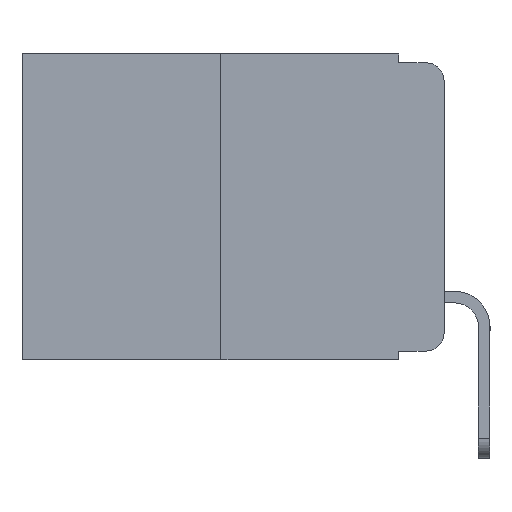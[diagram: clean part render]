
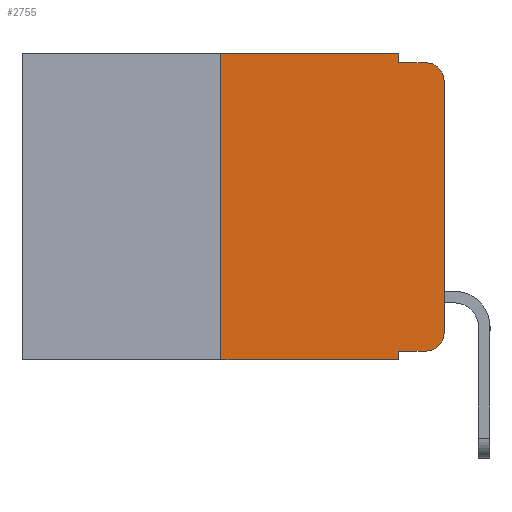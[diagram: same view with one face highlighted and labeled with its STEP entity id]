
A CAD part, left-side view. The second image highlights one B-rep face of the part: STEP entity #2755.
In plain terms, the highlighted planar face has unit normal (-1, 0, 0).
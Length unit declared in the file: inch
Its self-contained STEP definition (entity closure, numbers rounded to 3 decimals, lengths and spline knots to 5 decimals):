
#52 = EDGE_LOOP ( 'NONE', ( #12874, #5907, #13271, #6092, #5603, #7605, #6433, #11497, #13765, #5686 ) ) ;
#112 = DIRECTION ( 'NONE',  ( 0., -1., 0. ) ) ;
#180 = DIRECTION ( 'NONE',  ( -1., 0., 0. ) ) ;
#363 = VERTEX_POINT ( 'NONE', #12817 ) ;
#696 = VERTEX_POINT ( 'NONE', #8102 ) ;
#709 = DIRECTION ( 'NONE',  ( 0., 0., 1. ) ) ;
#1268 = DIRECTION ( 'NONE',  ( 0., 0., -1. ) ) ;
#1336 = CIRCLE ( 'NONE', #10804, 0.02 ) ;
#1537 = VECTOR ( 'NONE', #11410, 39.37008 ) ;
#1791 = VECTOR ( 'NONE', #3178, 39.37008 ) ;
#1844 = CARTESIAN_POINT ( 'NONE',  ( 0., 0.25, 0. ) ) ;
#2225 = VECTOR ( 'NONE', #6488, 39.37008 ) ;
#2282 = VERTEX_POINT ( 'NONE', #8865 ) ;
#2755 = ADVANCED_FACE ( 'NONE', ( #12239 ), #7552, .F. ) ;
#2836 = VERTEX_POINT ( 'NONE', #5837 ) ;
#3178 = DIRECTION ( 'NONE',  ( 0., -1., 0. ) ) ;
#3479 = VERTEX_POINT ( 'NONE', #12626 ) ;
#3719 = CARTESIAN_POINT ( 'NONE',  ( 0., 0.25, -0.343 ) ) ;
#3824 = VERTEX_POINT ( 'NONE', #12003 ) ;
#4120 = CIRCLE ( 'NONE', #6635, 0.02 ) ;
#4322 = AXIS2_PLACEMENT_3D ( 'NONE', #6410, #10486, #1268 ) ;
#4832 = CARTESIAN_POINT ( 'NONE',  ( 0., 0.25, 0. ) ) ;
#5000 = LINE ( 'NONE', #8538, #1791 ) ;
#5401 = CARTESIAN_POINT ( 'NONE',  ( 0., 0.051, 0. ) ) ;
#5542 = CARTESIAN_POINT ( 'NONE',  ( 0., 0.02, -0.03 ) ) ;
#5603 = ORIENTED_EDGE ( 'NONE', *, *, #14523, .F. ) ;
#5686 = ORIENTED_EDGE ( 'NONE', *, *, #11915, .T. ) ;
#5837 = CARTESIAN_POINT ( 'NONE',  ( 0., 0., -0.313 ) ) ;
#5885 = VERTEX_POINT ( 'NONE', #7036 ) ;
#5907 = ORIENTED_EDGE ( 'NONE', *, *, #12143, .T. ) ;
#6092 = ORIENTED_EDGE ( 'NONE', *, *, #12069, .F. ) ;
#6410 = CARTESIAN_POINT ( 'NONE',  ( 0., 0.473, 0. ) ) ;
#6433 = ORIENTED_EDGE ( 'NONE', *, *, #13144, .T. ) ;
#6488 = DIRECTION ( 'NONE',  ( 0., 0., -1. ) ) ;
#6495 = LINE ( 'NONE', #10785, #14507 ) ;
#6615 = DIRECTION ( 'NONE',  ( 0., 0., -1. ) ) ;
#6635 = AXIS2_PLACEMENT_3D ( 'NONE', #7350, #180, #8441 ) ;
#6946 = LINE ( 'NONE', #12173, #10099 ) ;
#7036 = CARTESIAN_POINT ( 'NONE',  ( 0., 0.051, -0.333 ) ) ;
#7205 = CARTESIAN_POINT ( 'NONE',  ( 0., 0.473, 0. ) ) ;
#7350 = CARTESIAN_POINT ( 'NONE',  ( 0., 0.02, -0.313 ) ) ;
#7552 = PLANE ( 'NONE',  #4322 ) ;
#7605 = ORIENTED_EDGE ( 'NONE', *, *, #12067, .F. ) ;
#8019 = DIRECTION ( 'NONE',  ( 0., -1., 0. ) ) ;
#8102 = CARTESIAN_POINT ( 'NONE',  ( 0., 0.051, -0.343 ) ) ;
#8165 = LINE ( 'NONE', #5401, #2225 ) ;
#8441 = DIRECTION ( 'NONE',  ( 0., 0., -1. ) ) ;
#8490 = VECTOR ( 'NONE', #10625, 39.37008 ) ;
#8538 = CARTESIAN_POINT ( 'NONE',  ( 0., 0.051, -0.01 ) ) ;
#8814 = VERTEX_POINT ( 'NONE', #4832 ) ;
#8865 = CARTESIAN_POINT ( 'NONE',  ( 0., 0., -0.03 ) ) ;
#9147 = VECTOR ( 'NONE', #13629, 39.37008 ) ;
#9493 = VECTOR ( 'NONE', #112, 39.37008 ) ;
#9953 = VERTEX_POINT ( 'NONE', #3719 ) ;
#10099 = VECTOR ( 'NONE', #8019, 39.37008 ) ;
#10387 = LINE ( 'NONE', #7205, #1537 ) ;
#10486 = DIRECTION ( 'NONE',  ( 1., 0., 0. ) ) ;
#10625 = DIRECTION ( 'NONE',  ( 0., 0., 1. ) ) ;
#10785 = CARTESIAN_POINT ( 'NONE',  ( 0., 0., 0. ) ) ;
#10804 = AXIS2_PLACEMENT_3D ( 'NONE', #5542, #12816, #6615 ) ;
#11410 = DIRECTION ( 'NONE',  ( 0., -1., 0. ) ) ;
#11497 = ORIENTED_EDGE ( 'NONE', *, *, #11958, .F. ) ;
#11838 = LINE ( 'NONE', #12547, #9147 ) ;
#11915 = EDGE_CURVE ( 'NONE', #3479, #2836, #4120, .T. ) ;
#11917 = EDGE_CURVE ( 'NONE', #5885, #3479, #12492, .T. ) ;
#11958 = EDGE_CURVE ( 'NONE', #5885, #696, #11838, .T. ) ;
#12003 = CARTESIAN_POINT ( 'NONE',  ( 0., 0.051, 0. ) ) ;
#12067 = EDGE_CURVE ( 'NONE', #9953, #8814, #13664, .T. ) ;
#12069 = EDGE_CURVE ( 'NONE', #3824, #363, #8165, .T. ) ;
#12087 = EDGE_CURVE ( 'NONE', #363, #13387, #5000, .T. ) ;
#12143 = EDGE_CURVE ( 'NONE', #2282, #13387, #1336, .T. ) ;
#12173 = CARTESIAN_POINT ( 'NONE',  ( 0., 0.473, -0.343 ) ) ;
#12194 = EDGE_CURVE ( 'NONE', #2836, #2282, #6495, .T. ) ;
#12239 = FACE_OUTER_BOUND ( 'NONE', #52, .T. ) ;
#12441 = CARTESIAN_POINT ( 'NONE',  ( 0., 0.02, -0.01 ) ) ;
#12492 = LINE ( 'NONE', #13587, #9493 ) ;
#12547 = CARTESIAN_POINT ( 'NONE',  ( 0., 0.051, 0. ) ) ;
#12626 = CARTESIAN_POINT ( 'NONE',  ( 0., 0.02, -0.333 ) ) ;
#12816 = DIRECTION ( 'NONE',  ( -1., 0., 0. ) ) ;
#12817 = CARTESIAN_POINT ( 'NONE',  ( 0., 0.051, -0.01 ) ) ;
#12874 = ORIENTED_EDGE ( 'NONE', *, *, #12194, .T. ) ;
#13144 = EDGE_CURVE ( 'NONE', #9953, #696, #6946, .T. ) ;
#13271 = ORIENTED_EDGE ( 'NONE', *, *, #12087, .F. ) ;
#13387 = VERTEX_POINT ( 'NONE', #12441 ) ;
#13587 = CARTESIAN_POINT ( 'NONE',  ( 0., 0.051, -0.333 ) ) ;
#13629 = DIRECTION ( 'NONE',  ( 0., 0., -1. ) ) ;
#13664 = LINE ( 'NONE', #1844, #8490 ) ;
#13765 = ORIENTED_EDGE ( 'NONE', *, *, #11917, .T. ) ;
#14507 = VECTOR ( 'NONE', #709, 39.37008 ) ;
#14523 = EDGE_CURVE ( 'NONE', #8814, #3824, #10387, .T. ) ;
